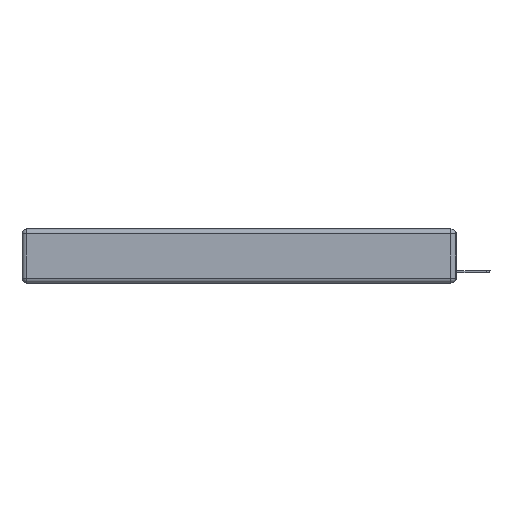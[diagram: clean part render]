
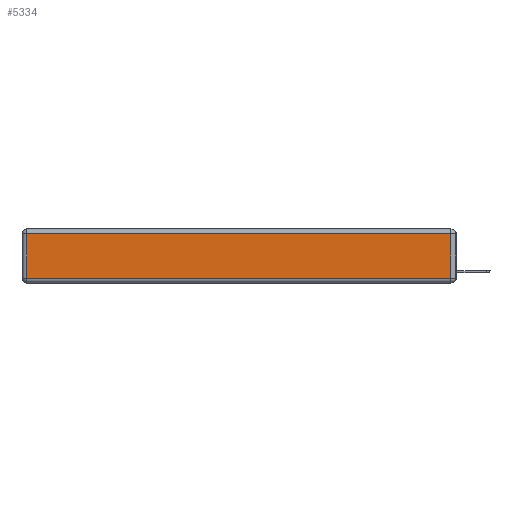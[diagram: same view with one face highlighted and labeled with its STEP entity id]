
A CAD part, left-side view. The second image highlights one B-rep face of the part: STEP entity #5334.
In plain terms, the highlighted planar face has unit normal (-1, 0, 0).
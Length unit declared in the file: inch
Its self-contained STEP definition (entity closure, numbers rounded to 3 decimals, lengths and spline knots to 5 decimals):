
#1573 = CARTESIAN_POINT ( 'NONE',  ( 0., 2.72, -0.313 ) ) ;
#1621 = VERTEX_POINT ( 'NONE', #1573 ) ;
#2218 = CARTESIAN_POINT ( 'NONE',  ( 0., 0.03, -0.343 ) ) ;
#3538 = EDGE_CURVE ( 'NONE', #1621, #7372, #10793, .T. ) ;
#3811 = VECTOR ( 'NONE', #14284, 39.37008 ) ;
#3913 = CARTESIAN_POINT ( 'NONE',  ( 0., 2.75, -0.03 ) ) ;
#4084 = VERTEX_POINT ( 'NONE', #15436 ) ;
#4139 = PLANE ( 'NONE',  #15494 ) ;
#4395 = VECTOR ( 'NONE', #12757, 39.37008 ) ;
#5083 = LINE ( 'NONE', #2218, #9696 ) ;
#5186 = EDGE_CURVE ( 'NONE', #7372, #4084, #5083, .T. ) ;
#5334 = ADVANCED_FACE ( 'NONE', ( #14557 ), #4139, .T. ) ;
#5562 = ORIENTED_EDGE ( 'NONE', *, *, #14953, .T. ) ;
#6607 = ORIENTED_EDGE ( 'NONE', *, *, #3538, .T. ) ;
#6637 = LINE ( 'NONE', #3913, #3811 ) ;
#7372 = VERTEX_POINT ( 'NONE', #11953 ) ;
#7849 = EDGE_LOOP ( 'NONE', ( #6607, #15990, #5562, #11809 ) ) ;
#7946 = CARTESIAN_POINT ( 'NONE',  ( 0., 2.72, -0.03 ) ) ;
#9266 = DIRECTION ( 'NONE',  ( -1., 0., 0. ) ) ;
#9318 = DIRECTION ( 'NONE',  ( 0., -1., 0. ) ) ;
#9696 = VECTOR ( 'NONE', #12551, 39.37008 ) ;
#10041 = LINE ( 'NONE', #12651, #4395 ) ;
#10559 = DIRECTION ( 'NONE',  ( 0., 0., 1. ) ) ;
#10793 = LINE ( 'NONE', #14458, #13627 ) ;
#11706 = CARTESIAN_POINT ( 'NONE',  ( 0., 0., -0.343 ) ) ;
#11809 = ORIENTED_EDGE ( 'NONE', *, *, #15423, .T. ) ;
#11953 = CARTESIAN_POINT ( 'NONE',  ( 0., 0.03, -0.313 ) ) ;
#12551 = DIRECTION ( 'NONE',  ( 0., 0., 1. ) ) ;
#12651 = CARTESIAN_POINT ( 'NONE',  ( 0., 2.72, -0.343 ) ) ;
#12757 = DIRECTION ( 'NONE',  ( 0., 0., -1. ) ) ;
#13627 = VECTOR ( 'NONE', #9318, 39.37008 ) ;
#14284 = DIRECTION ( 'NONE',  ( 0., 1., 0. ) ) ;
#14458 = CARTESIAN_POINT ( 'NONE',  ( 0., 0., -0.313 ) ) ;
#14557 = FACE_OUTER_BOUND ( 'NONE', #7849, .T. ) ;
#14953 = EDGE_CURVE ( 'NONE', #4084, #15654, #6637, .T. ) ;
#15423 = EDGE_CURVE ( 'NONE', #15654, #1621, #10041, .T. ) ;
#15436 = CARTESIAN_POINT ( 'NONE',  ( 0., 0.03, -0.03 ) ) ;
#15494 = AXIS2_PLACEMENT_3D ( 'NONE', #11706, #9266, #10559 ) ;
#15654 = VERTEX_POINT ( 'NONE', #7946 ) ;
#15990 = ORIENTED_EDGE ( 'NONE', *, *, #5186, .T. ) ;
